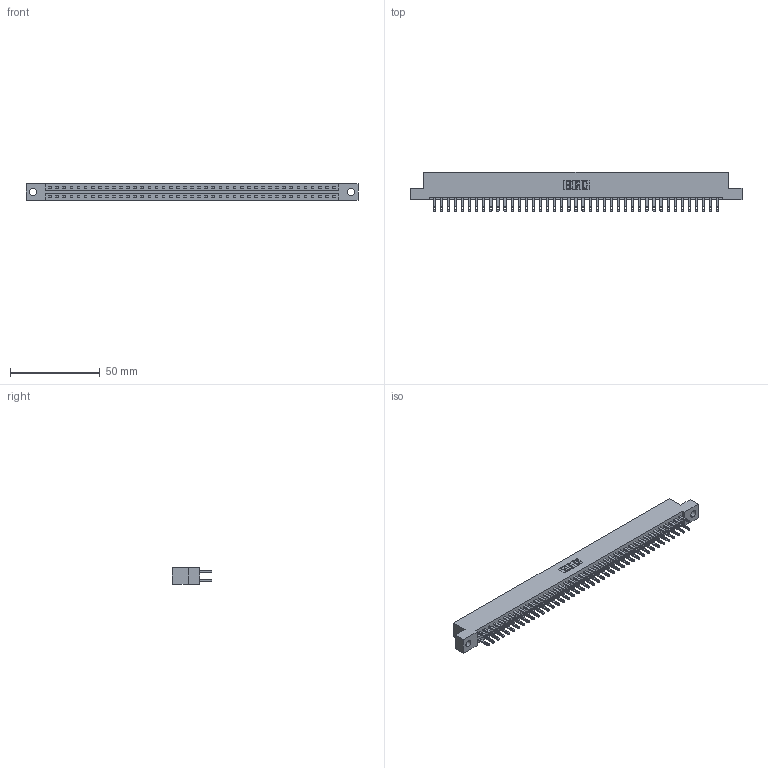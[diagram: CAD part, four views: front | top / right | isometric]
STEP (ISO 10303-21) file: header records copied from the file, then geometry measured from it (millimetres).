
FILE_DESCRIPTION (( 'STEP AP203' ), '1' );
FILE_NAME ('887-082-500-204.STEP', '2020-09-21T04:33:48', ( '' ), ( '' ), 'SwSTEP 2.0', 'SolidWorks 2020', '' );
FILE_SCHEMA (( 'CONFIG_CONTROL_DESIGN' ));
Length unit declared in the file: inch
Products named in the file (3): 887-082-500-204; 837 Part_Flush Mounting Lugs - 0.156 Dia-TH; 345-292-001_345-293-100
Assembly tree (83 placements, depth 2):
  887-082-500-204
    837 Part_Flush Mounting Lugs - 0.156 Dia-TH
    345-292-001_345-293-100  x82
Bounding box: 185.47 x 21.85 x 9.4 mm (x, y, z)
Volume: 19695.8 mm3; surface area: 22963.7 mm2
Topology: 83 solids, 83 shells, 4214 faces, 12857 edges, 8570 vertices
Faces by surface type: plane 2694, cylinder 1520
Entity records: 31851 total; most frequent: CARTESIAN_POINT 5366, ORIENTED_EDGE 5302, DIRECTION 4567, EDGE_CURVE 2651, LINE 2519, VECTOR 2519, VERTEX_POINT 1766, AXIS2_PLACEMENT_3D 1024
